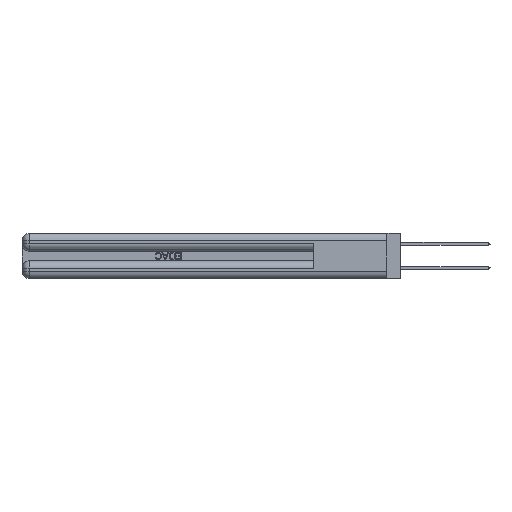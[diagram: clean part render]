
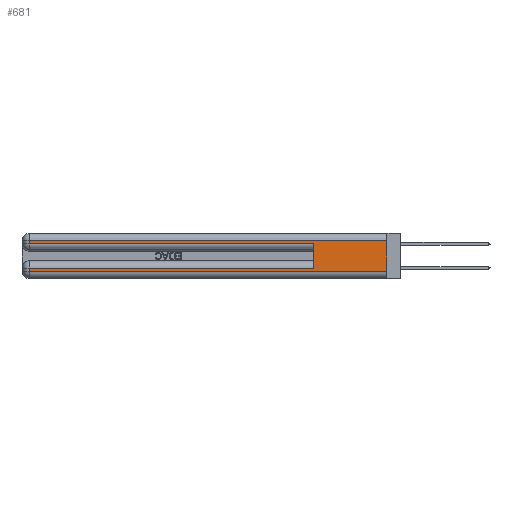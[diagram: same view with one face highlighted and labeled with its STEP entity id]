
A CAD part, left-side view. The second image highlights one B-rep face of the part: STEP entity #681.
In plain terms, the highlighted planar face has unit normal (-1, 0, 0).
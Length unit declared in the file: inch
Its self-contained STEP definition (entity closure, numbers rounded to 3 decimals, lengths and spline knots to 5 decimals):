
#681 = ADVANCED_FACE ( 'NONE', ( #22488 ), #23146, .F. ) ;
#788 = VERTEX_POINT ( 'NONE', #3059 ) ;
#2208 = LINE ( 'NONE', #16254, #44599 ) ;
#2524 = DIRECTION ( 'NONE',  ( 0., 0., -1. ) ) ;
#3059 = CARTESIAN_POINT ( 'NONE',  ( 0., 2.94, 0.31 ) ) ;
#3983 = VERTEX_POINT ( 'NONE', #5431 ) ;
#5235 = LINE ( 'NONE', #22717, #36766 ) ;
#5431 = CARTESIAN_POINT ( 'NONE',  ( 0., 0., 0.31 ) ) ;
#5498 = VECTOR ( 'NONE', #32257, 39.37008 ) ;
#11029 = EDGE_CURVE ( 'NONE', #23074, #39272, #15031, .T. ) ;
#11807 = EDGE_CURVE ( 'NONE', #33880, #45335, #41305, .T. ) ;
#12258 = CARTESIAN_POINT ( 'NONE',  ( 0., 0.6, 0.285 ) ) ;
#13057 = CARTESIAN_POINT ( 'NONE',  ( 0., 2.94, 0.085 ) ) ;
#13512 = LINE ( 'NONE', #35345, #23240 ) ;
#14574 = ORIENTED_EDGE ( 'NONE', *, *, #52225, .T. ) ;
#15031 = LINE ( 'NONE', #31389, #35612 ) ;
#15755 = ORIENTED_EDGE ( 'NONE', *, *, #11029, .T. ) ;
#16254 = CARTESIAN_POINT ( 'NONE',  ( 0., 0.6, 0.145 ) ) ;
#18624 = DIRECTION ( 'NONE',  ( 0., 0., -1. ) ) ;
#18894 = ORIENTED_EDGE ( 'NONE', *, *, #11807, .T. ) ;
#19629 = AXIS2_PLACEMENT_3D ( 'NONE', #51600, #27274, #2524 ) ;
#21658 = EDGE_CURVE ( 'NONE', #28269, #21969, #13512, .T. ) ;
#21969 = VERTEX_POINT ( 'NONE', #12258 ) ;
#22488 = FACE_OUTER_BOUND ( 'NONE', #23718, .T. ) ;
#22717 = CARTESIAN_POINT ( 'NONE',  ( 0., 2.94, 0.37 ) ) ;
#22734 = ORIENTED_EDGE ( 'NONE', *, *, #39133, .T. ) ;
#23074 = VERTEX_POINT ( 'NONE', #27008 ) ;
#23146 = PLANE ( 'NONE',  #19629 ) ;
#23240 = VECTOR ( 'NONE', #27300, 39.37008 ) ;
#23642 = ORIENTED_EDGE ( 'NONE', *, *, #48277, .F. ) ;
#23718 = EDGE_LOOP ( 'NONE', ( #23642, #25294, #14574, #39274, #33293, #18894, #22734, #15755 ) ) ;
#24562 = DIRECTION ( 'NONE',  ( 0., 0., 1. ) ) ;
#24742 = CARTESIAN_POINT ( 'NONE',  ( 0., 0.6, 0.085 ) ) ;
#25294 = ORIENTED_EDGE ( 'NONE', *, *, #27968, .T. ) ;
#27008 = CARTESIAN_POINT ( 'NONE',  ( 0., 2.94, 0.06 ) ) ;
#27274 = DIRECTION ( 'NONE',  ( 1., 0., 0. ) ) ;
#27300 = DIRECTION ( 'NONE',  ( 0., -1., 0. ) ) ;
#27968 = EDGE_CURVE ( 'NONE', #3983, #788, #46806, .T. ) ;
#28133 = CARTESIAN_POINT ( 'NONE',  ( 0., 0., 0.085 ) ) ;
#28269 = VERTEX_POINT ( 'NONE', #36553 ) ;
#31389 = CARTESIAN_POINT ( 'NONE',  ( 0., 0., 0.06 ) ) ;
#31665 = CARTESIAN_POINT ( 'NONE',  ( 0., 0., 0.06 ) ) ;
#32118 = LINE ( 'NONE', #39082, #44186 ) ;
#32257 = DIRECTION ( 'NONE',  ( 0., 0., -1. ) ) ;
#33293 = ORIENTED_EDGE ( 'NONE', *, *, #40604, .F. ) ;
#33880 = VERTEX_POINT ( 'NONE', #24742 ) ;
#35345 = CARTESIAN_POINT ( 'NONE',  ( 0., 0., 0.285 ) ) ;
#35484 = DIRECTION ( 'NONE',  ( 0., -1., 0. ) ) ;
#35612 = VECTOR ( 'NONE', #35484, 39.37008 ) ;
#36553 = CARTESIAN_POINT ( 'NONE',  ( 0., 2.94, 0.285 ) ) ;
#36766 = VECTOR ( 'NONE', #51183, 39.37008 ) ;
#38877 = CARTESIAN_POINT ( 'NONE',  ( 0., 0., 0.31 ) ) ;
#39082 = CARTESIAN_POINT ( 'NONE',  ( 0., 2.94, 0.37 ) ) ;
#39133 = EDGE_CURVE ( 'NONE', #45335, #23074, #5235, .T. ) ;
#39272 = VERTEX_POINT ( 'NONE', #31665 ) ;
#39274 = ORIENTED_EDGE ( 'NONE', *, *, #21658, .T. ) ;
#40604 = EDGE_CURVE ( 'NONE', #33880, #21969, #2208, .T. ) ;
#41305 = LINE ( 'NONE', #28133, #50802 ) ;
#42945 = DIRECTION ( 'NONE',  ( 0., 1., 0. ) ) ;
#44186 = VECTOR ( 'NONE', #18624, 39.37008 ) ;
#44599 = VECTOR ( 'NONE', #24562, 39.37008 ) ;
#45335 = VERTEX_POINT ( 'NONE', #13057 ) ;
#45545 = VECTOR ( 'NONE', #42945, 39.37008 ) ;
#46806 = LINE ( 'NONE', #38877, #45545 ) ;
#48277 = EDGE_CURVE ( 'NONE', #3983, #39272, #49045, .T. ) ;
#49045 = LINE ( 'NONE', #52479, #5498 ) ;
#50802 = VECTOR ( 'NONE', #52628, 39.37008 ) ;
#51183 = DIRECTION ( 'NONE',  ( 0., 0., -1. ) ) ;
#51600 = CARTESIAN_POINT ( 'NONE',  ( 0., 0., 0.37 ) ) ;
#52225 = EDGE_CURVE ( 'NONE', #788, #28269, #32118, .T. ) ;
#52479 = CARTESIAN_POINT ( 'NONE',  ( 0., 0., 0.37 ) ) ;
#52628 = DIRECTION ( 'NONE',  ( 0., 1., 0. ) ) ;
